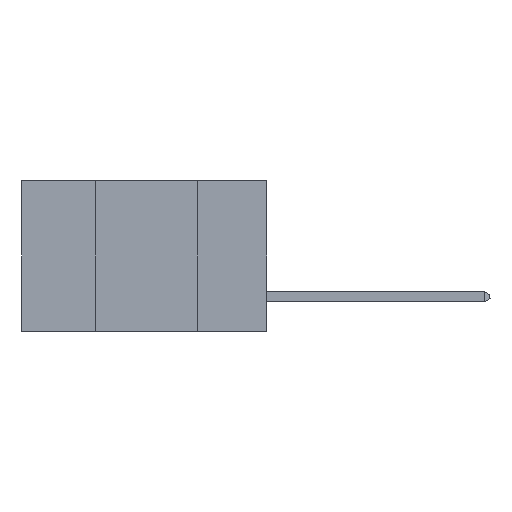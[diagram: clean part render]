
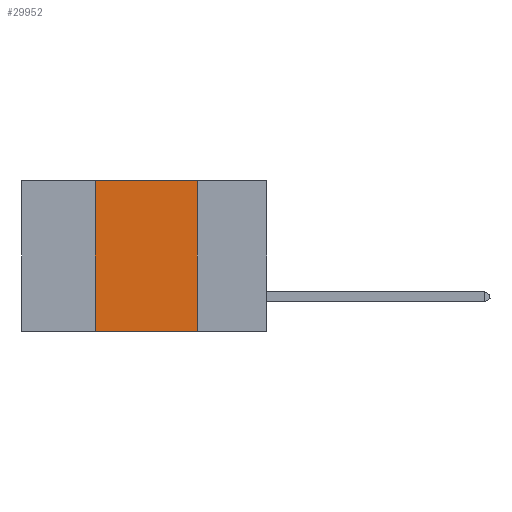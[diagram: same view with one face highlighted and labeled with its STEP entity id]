
A CAD part, left-side view. The second image highlights one B-rep face of the part: STEP entity #29952.
In plain terms, the highlighted planar face has unit normal (-1, 0, 0).
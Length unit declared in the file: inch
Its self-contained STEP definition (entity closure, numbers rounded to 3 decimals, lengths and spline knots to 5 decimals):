
#145 = VECTOR ( 'NONE', #8232, 39.37008 ) ;
#948 = EDGE_CURVE ( 'NONE', #38287, #22537, #7711, .T. ) ;
#4139 = DIRECTION ( 'NONE',  ( 0., 0., 1. ) ) ;
#7086 = CARTESIAN_POINT ( 'NONE',  ( 0., 0.17, 0. ) ) ;
#7711 = LINE ( 'NONE', #37018, #12470 ) ;
#7775 = AXIS2_PLACEMENT_3D ( 'NONE', #25438, #22340, #25733 ) ;
#8232 = DIRECTION ( 'NONE',  ( 0., -1., 0. ) ) ;
#10351 = DIRECTION ( 'NONE',  ( 0., -1., 0. ) ) ;
#11335 = VECTOR ( 'NONE', #19445, 39.37008 ) ;
#12470 = VECTOR ( 'NONE', #4139, 39.37008 ) ;
#17499 = CARTESIAN_POINT ( 'NONE',  ( 0., 0.17, -0.37 ) ) ;
#18643 = PLANE ( 'NONE',  #7775 ) ;
#19178 = LINE ( 'NONE', #20753, #20186 ) ;
#19445 = DIRECTION ( 'NONE',  ( 0., 0., -1. ) ) ;
#19805 = ORIENTED_EDGE ( 'NONE', *, *, #30176, .T. ) ;
#20067 = EDGE_CURVE ( 'NONE', #39613, #26517, #28158, .T. ) ;
#20186 = VECTOR ( 'NONE', #10351, 39.37008 ) ;
#20753 = CARTESIAN_POINT ( 'NONE',  ( 0., 0.6, -0.37 ) ) ;
#21313 = CARTESIAN_POINT ( 'NONE',  ( 0., 0.6, 0. ) ) ;
#22340 = DIRECTION ( 'NONE',  ( 1., 0., 0. ) ) ;
#22537 = VERTEX_POINT ( 'NONE', #40934 ) ;
#25393 = CARTESIAN_POINT ( 'NONE',  ( 0., 0.42, -0.37 ) ) ;
#25438 = CARTESIAN_POINT ( 'NONE',  ( 0., 0.6, 0. ) ) ;
#25733 = DIRECTION ( 'NONE',  ( 0., 0., -1. ) ) ;
#26233 = EDGE_CURVE ( 'NONE', #22537, #39613, #42791, .T. ) ;
#26517 = VERTEX_POINT ( 'NONE', #17499 ) ;
#28158 = LINE ( 'NONE', #42945, #11335 ) ;
#28362 = EDGE_LOOP ( 'NONE', ( #42528, #37562, #29456, #19805 ) ) ;
#29456 = ORIENTED_EDGE ( 'NONE', *, *, #948, .F. ) ;
#29952 = ADVANCED_FACE ( 'NONE', ( #32896 ), #18643, .F. ) ;
#30176 = EDGE_CURVE ( 'NONE', #38287, #26517, #19178, .T. ) ;
#32896 = FACE_OUTER_BOUND ( 'NONE', #28362, .T. ) ;
#37018 = CARTESIAN_POINT ( 'NONE',  ( 0., 0.42, 0. ) ) ;
#37562 = ORIENTED_EDGE ( 'NONE', *, *, #26233, .F. ) ;
#38287 = VERTEX_POINT ( 'NONE', #25393 ) ;
#39613 = VERTEX_POINT ( 'NONE', #7086 ) ;
#40934 = CARTESIAN_POINT ( 'NONE',  ( 0., 0.42, 0. ) ) ;
#42528 = ORIENTED_EDGE ( 'NONE', *, *, #20067, .F. ) ;
#42791 = LINE ( 'NONE', #21313, #145 ) ;
#42945 = CARTESIAN_POINT ( 'NONE',  ( 0., 0.17, 0. ) ) ;
